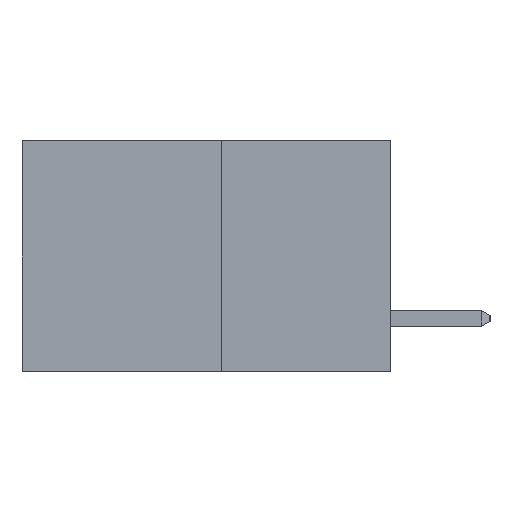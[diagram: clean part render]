
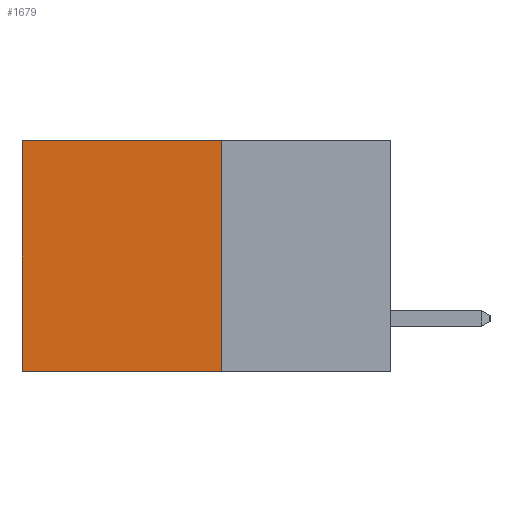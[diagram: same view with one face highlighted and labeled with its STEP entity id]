
A CAD part, left-side view. The second image highlights one B-rep face of the part: STEP entity #1679.
In plain terms, the highlighted planar face has unit normal (-1, 0, 0).
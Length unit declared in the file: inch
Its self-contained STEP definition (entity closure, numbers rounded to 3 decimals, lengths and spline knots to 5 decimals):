
#141 = CARTESIAN_POINT ( 'NONE',  ( 0.277, 0.27, -0.37 ) ) ;
#173 = DIRECTION ( 'NONE',  ( 1., 0., 0. ) ) ;
#547 = DIRECTION ( 'NONE',  ( 0., 1., 0. ) ) ;
#576 = DIRECTION ( 'NONE',  ( 0., 0., -1. ) ) ;
#1679 = ADVANCED_FACE ( 'NONE', ( #6462 ), #5769, .F. ) ;
#2006 = ORIENTED_EDGE ( 'NONE', *, *, #2176, .T. ) ;
#2087 = VECTOR ( 'NONE', #547, 39.37008 ) ;
#2176 = EDGE_CURVE ( 'NONE', #3070, #8608, #8664, .T. ) ;
#2458 = CARTESIAN_POINT ( 'NONE',  ( 0.277, 0.59, -0.37 ) ) ;
#3070 = VERTEX_POINT ( 'NONE', #5662 ) ;
#3086 = CARTESIAN_POINT ( 'NONE',  ( 0.277, 0.27, -0.37 ) ) ;
#3138 = EDGE_CURVE ( 'NONE', #4135, #6409, #8440, .T. ) ;
#3471 = AXIS2_PLACEMENT_3D ( 'NONE', #141, #173, #576 ) ;
#3941 = LINE ( 'NONE', #3086, #9442 ) ;
#4135 = VERTEX_POINT ( 'NONE', #5518 ) ;
#4190 = ORIENTED_EDGE ( 'NONE', *, *, #9047, .F. ) ;
#4215 = CARTESIAN_POINT ( 'NONE',  ( 0.277, 0.27, -0.37 ) ) ;
#4706 = CARTESIAN_POINT ( 'NONE',  ( 0.277, 0.59, -0.37 ) ) ;
#4874 = EDGE_CURVE ( 'NONE', #8608, #6409, #7885, .T. ) ;
#4877 = CARTESIAN_POINT ( 'NONE',  ( 0.277, 0.59, 0. ) ) ;
#5042 = EDGE_LOOP ( 'NONE', ( #6091, #8380, #4190, #2006 ) ) ;
#5518 = CARTESIAN_POINT ( 'NONE',  ( 0.277, 0.27, -0.37 ) ) ;
#5561 = DIRECTION ( 'NONE',  ( 0., 1., 0. ) ) ;
#5642 = VECTOR ( 'NONE', #6283, 39.37008 ) ;
#5662 = CARTESIAN_POINT ( 'NONE',  ( 0.277, 0.27, 0. ) ) ;
#5769 = PLANE ( 'NONE',  #3471 ) ;
#6091 = ORIENTED_EDGE ( 'NONE', *, *, #4874, .T. ) ;
#6283 = DIRECTION ( 'NONE',  ( 0., 0., -1. ) ) ;
#6409 = VERTEX_POINT ( 'NONE', #4706 ) ;
#6462 = FACE_OUTER_BOUND ( 'NONE', #5042, .T. ) ;
#7675 = DIRECTION ( 'NONE',  ( 0., 0., -1. ) ) ;
#7885 = LINE ( 'NONE', #2458, #5642 ) ;
#8268 = CARTESIAN_POINT ( 'NONE',  ( 0.277, 0.27, 0. ) ) ;
#8380 = ORIENTED_EDGE ( 'NONE', *, *, #3138, .F. ) ;
#8440 = LINE ( 'NONE', #4215, #2087 ) ;
#8454 = VECTOR ( 'NONE', #5561, 39.37008 ) ;
#8608 = VERTEX_POINT ( 'NONE', #4877 ) ;
#8664 = LINE ( 'NONE', #8268, #8454 ) ;
#9047 = EDGE_CURVE ( 'NONE', #3070, #4135, #3941, .T. ) ;
#9442 = VECTOR ( 'NONE', #7675, 39.37008 ) ;
